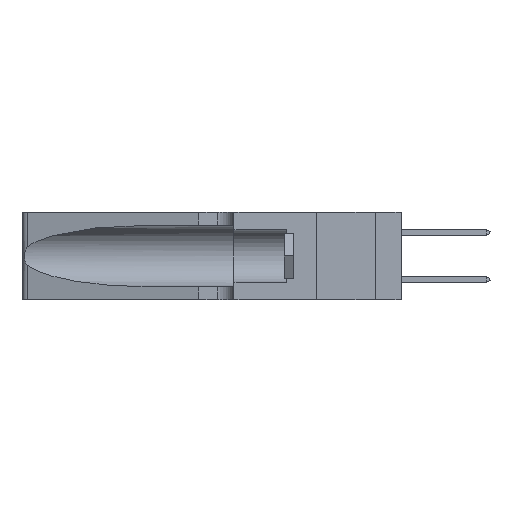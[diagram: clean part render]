
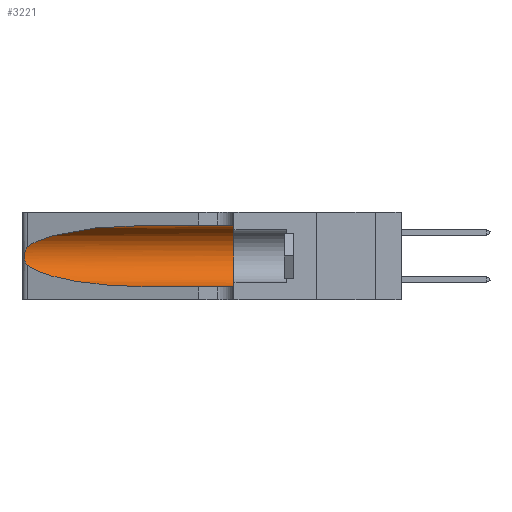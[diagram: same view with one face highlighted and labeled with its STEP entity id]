
A CAD part, left-side view. The second image highlights one B-rep face of the part: STEP entity #3221.
In plain terms, the highlighted cylindrical face has radius 3.308 mm (diameter 6.617 mm), a partial arc.
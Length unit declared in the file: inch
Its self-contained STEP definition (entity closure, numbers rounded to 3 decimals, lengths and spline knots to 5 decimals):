
#83 = CARTESIAN_POINT ( 'NONE',  ( 0.18966, 0.96281, 0.05475 ) ) ;
#240 = VERTEX_POINT ( 'NONE', #17725 ) ;
#1418 = ORIENTED_EDGE ( 'NONE', *, *, #35510, .F. ) ;
#1438 = DIRECTION ( 'NONE',  ( 0., -1., 0. ) ) ;
#2302 = CARTESIAN_POINT ( 'NONE',  ( 0.25487, 1.22718, 0.22369 ) ) ;
#2452 = CARTESIAN_POINT ( 'NONE',  ( 0.26017, 1.23833, 0.17102 ) ) ;
#2811 = VERTEX_POINT ( 'NONE', #13167 ) ;
#2947 = CARTESIAN_POINT ( 'NONE',  ( 0.1305, 0.72297, 0.31525 ) ) ;
#3221 = ADVANCED_FACE ( 'NONE', ( #29605 ), #37386, .F. ) ;
#5430 = VERTEX_POINT ( 'NONE', #36182 ) ;
#5679 = ORIENTED_EDGE ( 'NONE', *, *, #43271, .T. ) ;
#5910 = CARTESIAN_POINT ( 'NONE',  ( 0.25789, 1.23486, 0.15765 ) ) ;
#7461 = VERTEX_POINT ( 'NONE', #39559 ) ;
#7700 =( BOUNDED_CURVE ( )  B_SPLINE_CURVE ( 3, ( #40560, #37226, #83, #23959 ),
 .UNSPECIFIED., .F., .F. ) 
 B_SPLINE_CURVE_WITH_KNOTS ( ( 4, 4 ),
 ( 3.44316, 4.71239 ),
 .UNSPECIFIED. ) 
 CURVE ( )  GEOMETRIC_REPRESENTATION_ITEM ( )  RATIONAL_B_SPLINE_CURVE ( ( 1., 0.87, 0.87, 1. ) ) 
 REPRESENTATION_ITEM ( '' )  );
#9369 = CARTESIAN_POINT ( 'NONE',  ( 0.25555, 1.22993, 0.14849 ) ) ;
#9875 = CARTESIAN_POINT ( 'NONE',  ( 0.18966, 0.96281, 0.31525 ) ) ;
#10415 = CARTESIAN_POINT ( 'NONE',  ( 0.1305, 0.72297, 0.05475 ) ) ;
#10554 = AXIS2_PLACEMENT_3D ( 'NONE', #21870, #1438, #41835 ) ;
#12001 = VERTEX_POINT ( 'NONE', #15906 ) ;
#12720 = EDGE_CURVE ( 'NONE', #7461, #21281, #7700, .T. ) ;
#13167 = CARTESIAN_POINT ( 'NONE',  ( 0.1305, 0.35, 0.31525 ) ) ;
#14510 = CARTESIAN_POINT ( 'NONE',  ( 0.1305, 0.35, 0.185 ) ) ;
#15906 = CARTESIAN_POINT ( 'NONE',  ( 0.25487, 1.22718, 0.22369 ) ) ;
#16049 = CARTESIAN_POINT ( 'NONE',  ( 0.25787, 1.23484, 0.2124 ) ) ;
#16402 = LINE ( 'NONE', #39941, #33206 ) ;
#17120 = VECTOR ( 'NONE', #35892, 39.37008 ) ;
#17593 = CIRCLE ( 'NONE', #41125, 0.13025 ) ;
#17725 = CARTESIAN_POINT ( 'NONE',  ( 0.1305, 0.72297, 0.31525 ) ) ;
#17918 = DIRECTION ( 'NONE',  ( 0., 0., 1. ) ) ;
#17971 = ORIENTED_EDGE ( 'NONE', *, *, #36816, .F. ) ;
#19482 = CARTESIAN_POINT ( 'NONE',  ( 0.26018, 1.23835, 0.19895 ) ) ;
#20113 = CARTESIAN_POINT ( 'NONE',  ( 0.2373, 1.15595, 0.28018 ) ) ;
#21281 = VERTEX_POINT ( 'NONE', #10415 ) ;
#21870 = CARTESIAN_POINT ( 'NONE',  ( 0.1305, 1.61858, 0.185 ) ) ;
#22855 = CARTESIAN_POINT ( 'NONE',  ( 0.26075, 1.23896, 0.178 ) ) ;
#23959 = CARTESIAN_POINT ( 'NONE',  ( 0.1305, 0.72297, 0.05475 ) ) ;
#24521 = EDGE_CURVE ( 'NONE', #21281, #5430, #16402, .T. ) ;
#24824 =( BOUNDED_CURVE ( )  B_SPLINE_CURVE ( 3, ( #2947, #9875, #20113, #43466 ),
 .UNSPECIFIED., .F., .F. ) 
 B_SPLINE_CURVE_WITH_KNOTS ( ( 4, 4 ),
 ( 1.5708, 2.84003 ),
 .UNSPECIFIED. ) 
 CURVE ( )  GEOMETRIC_REPRESENTATION_ITEM ( )  RATIONAL_B_SPLINE_CURVE ( ( 1., 0.87, 0.87, 1. ) ) 
 REPRESENTATION_ITEM ( '' )  );
#24862 = ORIENTED_EDGE ( 'NONE', *, *, #12720, .T. ) ;
#25434 = ORIENTED_EDGE ( 'NONE', *, *, #24521, .T. ) ;
#26085 = LINE ( 'NONE', #32526, #17120 ) ;
#26232 = CARTESIAN_POINT ( 'NONE',  ( 0.25856, 1.23593, 0.16098 ) ) ;
#28421 = EDGE_LOOP ( 'NONE', ( #5679, #37343, #24862, #25434, #17971, #1418 ) ) ;
#29602 = CARTESIAN_POINT ( 'NONE',  ( 0.25639, 1.23186, 0.15144 ) ) ;
#29605 = FACE_OUTER_BOUND ( 'NONE', #28421, .T. ) ;
#32526 = CARTESIAN_POINT ( 'NONE',  ( 0.1305, 1.61858, 0.31525 ) ) ;
#32928 = CARTESIAN_POINT ( 'NONE',  ( 0.25487, 1.22718, 0.14631 ) ) ;
#33206 = VECTOR ( 'NONE', #39791, 39.37008 ) ;
#35510 = EDGE_CURVE ( 'NONE', #240, #2811, #26085, .T. ) ;
#35892 = DIRECTION ( 'NONE',  ( 0., -1., 0. ) ) ;
#36079 = EDGE_CURVE ( 'NONE', #12001, #7461, #40283, .T. ) ;
#36148 = CARTESIAN_POINT ( 'NONE',  ( 0.25639, 1.23184, 0.21858 ) ) ;
#36182 = CARTESIAN_POINT ( 'NONE',  ( 0.1305, 0.35, 0.05475 ) ) ;
#36816 = EDGE_CURVE ( 'NONE', #2811, #5430, #17593, .T. ) ;
#37226 = CARTESIAN_POINT ( 'NONE',  ( 0.2373, 1.15595, 0.08982 ) ) ;
#37343 = ORIENTED_EDGE ( 'NONE', *, *, #36079, .T. ) ;
#37386 = CYLINDRICAL_SURFACE ( 'NONE', #10554, 0.13025 ) ;
#37936 = DIRECTION ( 'NONE',  ( 0., 1., 0. ) ) ;
#39465 = CARTESIAN_POINT ( 'NONE',  ( 0.25854, 1.2359, 0.20912 ) ) ;
#39559 = CARTESIAN_POINT ( 'NONE',  ( 0.25487, 1.22718, 0.14631 ) ) ;
#39791 = DIRECTION ( 'NONE',  ( 0., -1., 0. ) ) ;
#39941 = CARTESIAN_POINT ( 'NONE',  ( 0.1305, 1.61858, 0.05475 ) ) ;
#40283 = B_SPLINE_CURVE_WITH_KNOTS ( 'NONE', 3,
 ( #2302, #42690, #36148, #16049, #39465, #19482, #42830, #22855, #2452, #26232, #5910, #29602, #9369, #32928 ),
 .UNSPECIFIED., .F., .F.,
 ( 4, 2, 2, 2, 2, 2, 4 ),
 ( 0., 0.00027, 0.00053, 0.00107, 0.0016, 0.00187, 0.00214 ),
 .UNSPECIFIED. ) ;
#40560 = CARTESIAN_POINT ( 'NONE',  ( 0.25487, 1.22718, 0.14631 ) ) ;
#41125 = AXIS2_PLACEMENT_3D ( 'NONE', #14510, #37936, #17918 ) ;
#41835 = DIRECTION ( 'NONE',  ( 0., 0., -1. ) ) ;
#42690 = CARTESIAN_POINT ( 'NONE',  ( 0.25555, 1.22994, 0.2215 ) ) ;
#42830 = CARTESIAN_POINT ( 'NONE',  ( 0.26075, 1.23896, 0.19203 ) ) ;
#43271 = EDGE_CURVE ( 'NONE', #240, #12001, #24824, .T. ) ;
#43466 = CARTESIAN_POINT ( 'NONE',  ( 0.25487, 1.22718, 0.22369 ) ) ;
